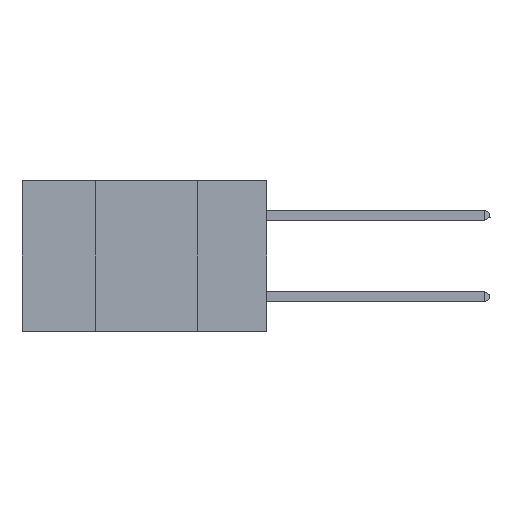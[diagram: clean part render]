
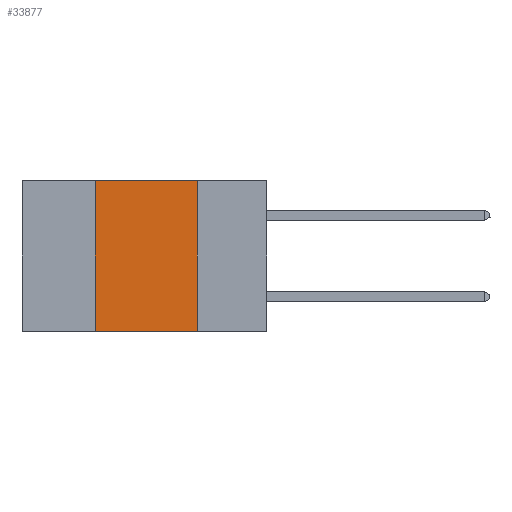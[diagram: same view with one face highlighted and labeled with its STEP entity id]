
A CAD part, left-side view. The second image highlights one B-rep face of the part: STEP entity #33877.
In plain terms, the highlighted planar face has unit normal (-1, 0, 0).
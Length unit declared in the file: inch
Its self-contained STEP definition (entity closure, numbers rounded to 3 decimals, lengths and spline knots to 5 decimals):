
#2110 = VECTOR ( 'NONE', #10241, 39.37008 ) ;
#2699 = CARTESIAN_POINT ( 'NONE',  ( 0., 0.6, 0. ) ) ;
#5645 = CARTESIAN_POINT ( 'NONE',  ( 0., 0.42, 0. ) ) ;
#5650 = LINE ( 'NONE', #19604, #20484 ) ;
#5657 = FACE_OUTER_BOUND ( 'NONE', #24238, .T. ) ;
#5663 = CARTESIAN_POINT ( 'NONE',  ( 0., 0.42, 0. ) ) ;
#6158 = LINE ( 'NONE', #2699, #38923 ) ;
#10052 = VERTEX_POINT ( 'NONE', #14774 ) ;
#10241 = DIRECTION ( 'NONE',  ( 0., -1., 0. ) ) ;
#11165 = EDGE_CURVE ( 'NONE', #25201, #35220, #26511, .T. ) ;
#12747 = ORIENTED_EDGE ( 'NONE', *, *, #26359, .T. ) ;
#13213 = CARTESIAN_POINT ( 'NONE',  ( 0., 0.6, 0. ) ) ;
#14585 = VECTOR ( 'NONE', #33161, 39.37008 ) ;
#14774 = CARTESIAN_POINT ( 'NONE',  ( 0., 0.17, 0. ) ) ;
#16449 = DIRECTION ( 'NONE',  ( 0., -1., 0. ) ) ;
#17984 = CARTESIAN_POINT ( 'NONE',  ( 0., 0.6, -0.37 ) ) ;
#19604 = CARTESIAN_POINT ( 'NONE',  ( 0., 0.17, 0. ) ) ;
#19848 = DIRECTION ( 'NONE',  ( 1., 0., 0. ) ) ;
#20484 = VECTOR ( 'NONE', #33598, 39.37008 ) ;
#21674 = CARTESIAN_POINT ( 'NONE',  ( 0., 0.17, -0.37 ) ) ;
#24238 = EDGE_LOOP ( 'NONE', ( #24316, #30958, #26063, #12747 ) ) ;
#24316 = ORIENTED_EDGE ( 'NONE', *, *, #29749, .F. ) ;
#25201 = VERTEX_POINT ( 'NONE', #39614 ) ;
#26063 = ORIENTED_EDGE ( 'NONE', *, *, #11165, .F. ) ;
#26359 = EDGE_CURVE ( 'NONE', #25201, #38350, #42281, .T. ) ;
#26511 = LINE ( 'NONE', #5663, #14585 ) ;
#26627 = AXIS2_PLACEMENT_3D ( 'NONE', #13213, #19848, #30377 ) ;
#29749 = EDGE_CURVE ( 'NONE', #10052, #38350, #5650, .T. ) ;
#30377 = DIRECTION ( 'NONE',  ( 0., 0., -1. ) ) ;
#30958 = ORIENTED_EDGE ( 'NONE', *, *, #32072, .F. ) ;
#32072 = EDGE_CURVE ( 'NONE', #35220, #10052, #6158, .T. ) ;
#33161 = DIRECTION ( 'NONE',  ( 0., 0., 1. ) ) ;
#33598 = DIRECTION ( 'NONE',  ( 0., 0., -1. ) ) ;
#33877 = ADVANCED_FACE ( 'NONE', ( #5657 ), #43911, .F. ) ;
#35220 = VERTEX_POINT ( 'NONE', #5645 ) ;
#38350 = VERTEX_POINT ( 'NONE', #21674 ) ;
#38923 = VECTOR ( 'NONE', #16449, 39.37008 ) ;
#39614 = CARTESIAN_POINT ( 'NONE',  ( 0., 0.42, -0.37 ) ) ;
#42281 = LINE ( 'NONE', #17984, #2110 ) ;
#43911 = PLANE ( 'NONE',  #26627 ) ;
